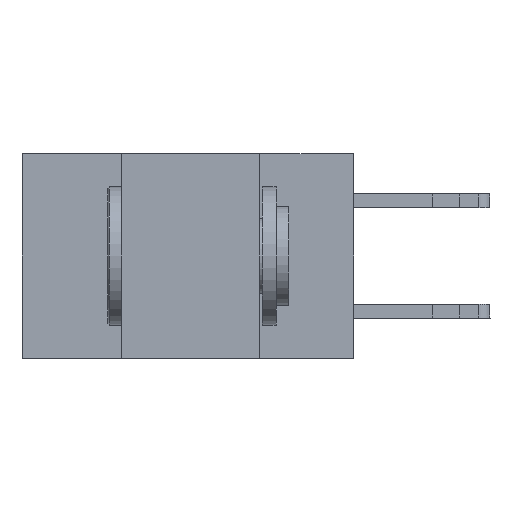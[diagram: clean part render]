
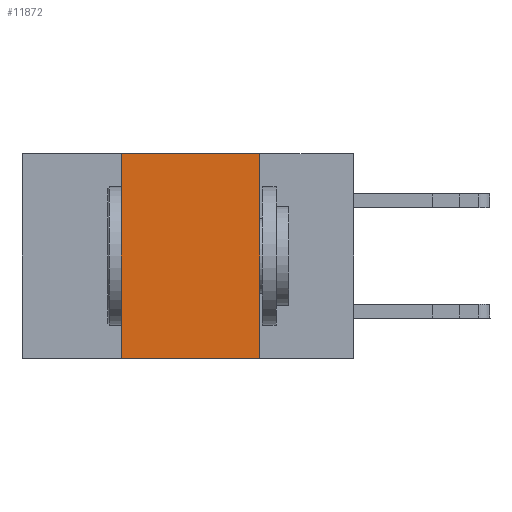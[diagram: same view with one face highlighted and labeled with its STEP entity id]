
A CAD part, left-side view. The second image highlights one B-rep face of the part: STEP entity #11872.
In plain terms, the highlighted planar face has unit normal (-1, 0, 0).
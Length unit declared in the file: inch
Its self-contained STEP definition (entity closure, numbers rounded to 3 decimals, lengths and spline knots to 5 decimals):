
#408 = FACE_OUTER_BOUND ( 'NONE', #13841, .T. ) ;
#2675 = DIRECTION ( 'NONE',  ( 0., -1., 0. ) ) ;
#2990 = VECTOR ( 'NONE', #18849, 39.37008 ) ;
#3063 = CARTESIAN_POINT ( 'NONE',  ( 0., 0.6, 0. ) ) ;
#3085 = VERTEX_POINT ( 'NONE', #16832 ) ;
#3180 = VECTOR ( 'NONE', #2675, 39.37008 ) ;
#3195 = EDGE_CURVE ( 'NONE', #3085, #14033, #14950, .T. ) ;
#3719 = CARTESIAN_POINT ( 'NONE',  ( 0., 0.17, 0. ) ) ;
#4348 = EDGE_CURVE ( 'NONE', #14033, #7965, #10552, .T. ) ;
#4732 = DIRECTION ( 'NONE',  ( 1., 0., 0. ) ) ;
#5283 = LINE ( 'NONE', #3719, #13597 ) ;
#6014 = VERTEX_POINT ( 'NONE', #8274 ) ;
#7965 = VERTEX_POINT ( 'NONE', #18057 ) ;
#8274 = CARTESIAN_POINT ( 'NONE',  ( 0., 0.17, -0.37 ) ) ;
#9030 = AXIS2_PLACEMENT_3D ( 'NONE', #9427, #4732, #15650 ) ;
#9427 = CARTESIAN_POINT ( 'NONE',  ( 0., 0.6, 0. ) ) ;
#10538 = ORIENTED_EDGE ( 'NONE', *, *, #13274, .F. ) ;
#10552 = LINE ( 'NONE', #3063, #3180 ) ;
#11734 = CARTESIAN_POINT ( 'NONE',  ( 0., 0.42, 0. ) ) ;
#11872 = ADVANCED_FACE ( 'NONE', ( #408 ), #17041, .F. ) ;
#11988 = EDGE_CURVE ( 'NONE', #3085, #6014, #14057, .T. ) ;
#12371 = ORIENTED_EDGE ( 'NONE', *, *, #4348, .F. ) ;
#12847 = DIRECTION ( 'NONE',  ( 0., -1., 0. ) ) ;
#13274 = EDGE_CURVE ( 'NONE', #7965, #6014, #5283, .T. ) ;
#13577 = VECTOR ( 'NONE', #12847, 39.37008 ) ;
#13597 = VECTOR ( 'NONE', #14640, 39.37008 ) ;
#13841 = EDGE_LOOP ( 'NONE', ( #10538, #12371, #16175, #14068 ) ) ;
#14033 = VERTEX_POINT ( 'NONE', #11734 ) ;
#14057 = LINE ( 'NONE', #18903, #13577 ) ;
#14068 = ORIENTED_EDGE ( 'NONE', *, *, #11988, .T. ) ;
#14640 = DIRECTION ( 'NONE',  ( 0., 0., -1. ) ) ;
#14950 = LINE ( 'NONE', #16956, #2990 ) ;
#15650 = DIRECTION ( 'NONE',  ( 0., 0., -1. ) ) ;
#16175 = ORIENTED_EDGE ( 'NONE', *, *, #3195, .F. ) ;
#16832 = CARTESIAN_POINT ( 'NONE',  ( 0., 0.42, -0.37 ) ) ;
#16956 = CARTESIAN_POINT ( 'NONE',  ( 0., 0.42, 0. ) ) ;
#17041 = PLANE ( 'NONE',  #9030 ) ;
#18057 = CARTESIAN_POINT ( 'NONE',  ( 0., 0.17, 0. ) ) ;
#18849 = DIRECTION ( 'NONE',  ( 0., 0., 1. ) ) ;
#18903 = CARTESIAN_POINT ( 'NONE',  ( 0., 0.6, -0.37 ) ) ;
